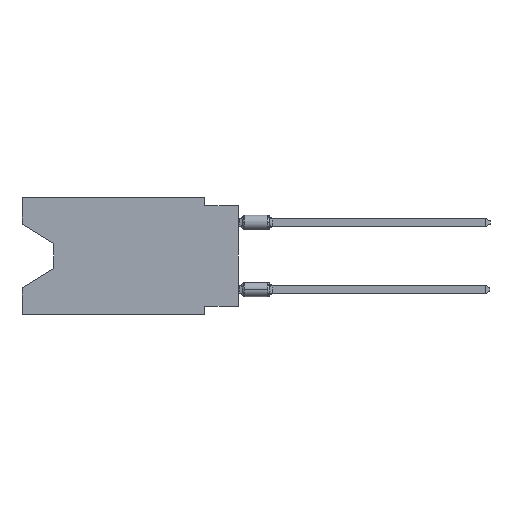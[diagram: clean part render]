
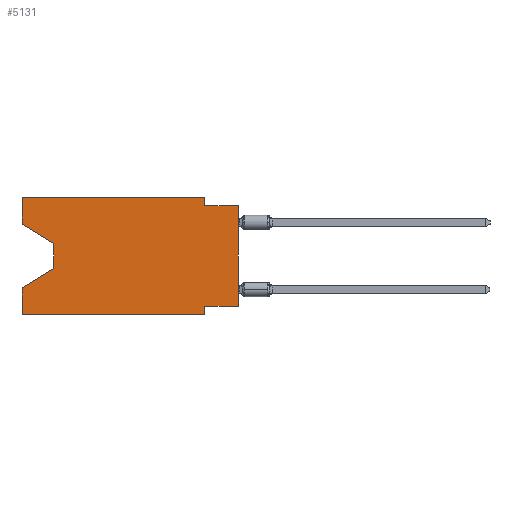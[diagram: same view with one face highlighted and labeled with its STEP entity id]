
A CAD part, left-side view. The second image highlights one B-rep face of the part: STEP entity #5131.
In plain terms, the highlighted planar face has unit normal (-1, 0, 0).
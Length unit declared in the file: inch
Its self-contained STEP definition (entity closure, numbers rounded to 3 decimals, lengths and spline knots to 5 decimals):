
#167 = VERTEX_POINT ( 'NONE', #13119 ) ;
#175 = CARTESIAN_POINT ( 'NONE',  ( 0., 0.55, -0.212 ) ) ;
#440 = EDGE_CURVE ( 'NONE', #2682, #5523, #7974, .T. ) ;
#651 = DIRECTION ( 'NONE',  ( 0., -1., 0. ) ) ;
#668 = VECTOR ( 'NONE', #1532, 39.37008 ) ;
#888 = ORIENTED_EDGE ( 'NONE', *, *, #7094, .T. ) ;
#942 = EDGE_CURVE ( 'NONE', #1382, #167, #12874, .T. ) ;
#992 = AXIS2_PLACEMENT_3D ( 'NONE', #11688, #10639, #1176 ) ;
#1126 = LINE ( 'NONE', #6563, #8957 ) ;
#1139 = ORIENTED_EDGE ( 'NONE', *, *, #942, .F. ) ;
#1176 = DIRECTION ( 'NONE',  ( 0., 0., -1. ) ) ;
#1268 = CARTESIAN_POINT ( 'NONE',  ( 0., 0.645, -0.35 ) ) ;
#1359 = CARTESIAN_POINT ( 'NONE',  ( 0., 0.1, -0.35 ) ) ;
#1382 = VERTEX_POINT ( 'NONE', #2612 ) ;
#1401 = VERTEX_POINT ( 'NONE', #12295 ) ;
#1532 = DIRECTION ( 'NONE',  ( 0., -1., 0. ) ) ;
#1541 = VECTOR ( 'NONE', #3650, 39.37008 ) ;
#1674 = DIRECTION ( 'NONE',  ( 0., 0., -1. ) ) ;
#1854 = ORIENTED_EDGE ( 'NONE', *, *, #4886, .T. ) ;
#1978 = ORIENTED_EDGE ( 'NONE', *, *, #6322, .F. ) ;
#2308 = VERTEX_POINT ( 'NONE', #2576 ) ;
#2365 = VECTOR ( 'NONE', #3681, 39.37008 ) ;
#2500 = CARTESIAN_POINT ( 'NONE',  ( 0., 0., -0.025 ) ) ;
#2503 = LINE ( 'NONE', #8784, #2365 ) ;
#2576 = CARTESIAN_POINT ( 'NONE',  ( 0., 0.55, -0.138 ) ) ;
#2612 = CARTESIAN_POINT ( 'NONE',  ( 0., 0.645, 0. ) ) ;
#2636 = DIRECTION ( 'NONE',  ( 0., -0.855, -0.519 ) ) ;
#2682 = VERTEX_POINT ( 'NONE', #1268 ) ;
#2880 = EDGE_CURVE ( 'NONE', #167, #10988, #10022, .T. ) ;
#2907 = EDGE_CURVE ( 'NONE', #9970, #5523, #13082, .T. ) ;
#3005 = CARTESIAN_POINT ( 'NONE',  ( 0., 0., -0.025 ) ) ;
#3046 = LINE ( 'NONE', #7107, #8913 ) ;
#3388 = CARTESIAN_POINT ( 'NONE',  ( 0., 0.645, 0. ) ) ;
#3650 = DIRECTION ( 'NONE',  ( 0., -1., 0. ) ) ;
#3681 = DIRECTION ( 'NONE',  ( 0., 0., -1. ) ) ;
#3987 = VERTEX_POINT ( 'NONE', #2500 ) ;
#4210 = EDGE_LOOP ( 'NONE', ( #888, #6647, #1854, #5149, #9001, #7618, #4676, #7232, #8996, #10984, #1139, #1978 ) ) ;
#4544 = VECTOR ( 'NONE', #5279, 39.37008 ) ;
#4676 = ORIENTED_EDGE ( 'NONE', *, *, #11320, .F. ) ;
#4796 = CARTESIAN_POINT ( 'NONE',  ( 0., 0.55, -0.212 ) ) ;
#4886 = EDGE_CURVE ( 'NONE', #6422, #8089, #7685, .T. ) ;
#5061 = EDGE_CURVE ( 'NONE', #11012, #3987, #3046, .T. ) ;
#5131 = ADVANCED_FACE ( 'NONE', ( #9665 ), #6404, .F. ) ;
#5149 = ORIENTED_EDGE ( 'NONE', *, *, #12013, .F. ) ;
#5279 = DIRECTION ( 'NONE',  ( 0., 0., 1. ) ) ;
#5523 = VERTEX_POINT ( 'NONE', #1359 ) ;
#5727 = LINE ( 'NONE', #7864, #11079 ) ;
#5821 = VECTOR ( 'NONE', #6702, 39.37008 ) ;
#6211 = CARTESIAN_POINT ( 'NONE',  ( 0., 0., -0.325 ) ) ;
#6322 = EDGE_CURVE ( 'NONE', #1401, #1382, #11880, .T. ) ;
#6404 = PLANE ( 'NONE',  #992 ) ;
#6422 = VERTEX_POINT ( 'NONE', #4796 ) ;
#6563 = CARTESIAN_POINT ( 'NONE',  ( 0., 0.645, -0.08025 ) ) ;
#6647 = ORIENTED_EDGE ( 'NONE', *, *, #9694, .T. ) ;
#6702 = DIRECTION ( 'NONE',  ( 0., 0., -1. ) ) ;
#6717 = VECTOR ( 'NONE', #1674, 39.37008 ) ;
#7094 = EDGE_CURVE ( 'NONE', #1401, #2308, #1126, .T. ) ;
#7107 = CARTESIAN_POINT ( 'NONE',  ( 0., 0., 0. ) ) ;
#7232 = ORIENTED_EDGE ( 'NONE', *, *, #5061, .T. ) ;
#7554 = VECTOR ( 'NONE', #8860, 39.37008 ) ;
#7597 = VECTOR ( 'NONE', #10817, 39.37008 ) ;
#7618 = ORIENTED_EDGE ( 'NONE', *, *, #2907, .F. ) ;
#7685 = LINE ( 'NONE', #175, #7597 ) ;
#7737 = CARTESIAN_POINT ( 'NONE',  ( 0., 0.1, 0. ) ) ;
#7864 = CARTESIAN_POINT ( 'NONE',  ( 0., 0., -0.325 ) ) ;
#7888 = LINE ( 'NONE', #11090, #7554 ) ;
#7974 = LINE ( 'NONE', #12299, #1541 ) ;
#8089 = VERTEX_POINT ( 'NONE', #13503 ) ;
#8094 = EDGE_CURVE ( 'NONE', #10988, #3987, #12470, .T. ) ;
#8784 = CARTESIAN_POINT ( 'NONE',  ( 0., 0.55, -0.138 ) ) ;
#8860 = DIRECTION ( 'NONE',  ( 0., 0., 1. ) ) ;
#8913 = VECTOR ( 'NONE', #12380, 39.37008 ) ;
#8957 = VECTOR ( 'NONE', #2636, 39.37008 ) ;
#8996 = ORIENTED_EDGE ( 'NONE', *, *, #8094, .F. ) ;
#9001 = ORIENTED_EDGE ( 'NONE', *, *, #440, .T. ) ;
#9665 = FACE_OUTER_BOUND ( 'NONE', #4210, .T. ) ;
#9694 = EDGE_CURVE ( 'NONE', #2308, #6422, #2503, .T. ) ;
#9735 = DIRECTION ( 'NONE',  ( 0., 1., 0. ) ) ;
#9970 = VERTEX_POINT ( 'NONE', #12038 ) ;
#10022 = LINE ( 'NONE', #7737, #5821 ) ;
#10639 = DIRECTION ( 'NONE',  ( 1., 0., 0. ) ) ;
#10817 = DIRECTION ( 'NONE',  ( 0., 0.855, -0.519 ) ) ;
#10836 = CARTESIAN_POINT ( 'NONE',  ( 0., 0.645, 0. ) ) ;
#10945 = VECTOR ( 'NONE', #651, 39.37008 ) ;
#10984 = ORIENTED_EDGE ( 'NONE', *, *, #2880, .F. ) ;
#10988 = VERTEX_POINT ( 'NONE', #12460 ) ;
#11012 = VERTEX_POINT ( 'NONE', #6211 ) ;
#11071 = CARTESIAN_POINT ( 'NONE',  ( 0., 0.1, -0.35 ) ) ;
#11079 = VECTOR ( 'NONE', #9735, 39.37008 ) ;
#11090 = CARTESIAN_POINT ( 'NONE',  ( 0., 0.645, 0. ) ) ;
#11320 = EDGE_CURVE ( 'NONE', #11012, #9970, #5727, .T. ) ;
#11688 = CARTESIAN_POINT ( 'NONE',  ( 0., 0.645, 0. ) ) ;
#11880 = LINE ( 'NONE', #10836, #4544 ) ;
#12013 = EDGE_CURVE ( 'NONE', #2682, #8089, #7888, .T. ) ;
#12038 = CARTESIAN_POINT ( 'NONE',  ( 0., 0.1, -0.325 ) ) ;
#12295 = CARTESIAN_POINT ( 'NONE',  ( 0., 0.645, -0.08025 ) ) ;
#12299 = CARTESIAN_POINT ( 'NONE',  ( 0., 0.645, -0.35 ) ) ;
#12380 = DIRECTION ( 'NONE',  ( 0., 0., 1. ) ) ;
#12460 = CARTESIAN_POINT ( 'NONE',  ( 0., 0.1, -0.025 ) ) ;
#12470 = LINE ( 'NONE', #3005, #10945 ) ;
#12874 = LINE ( 'NONE', #3388, #668 ) ;
#13082 = LINE ( 'NONE', #11071, #6717 ) ;
#13119 = CARTESIAN_POINT ( 'NONE',  ( 0., 0.1, 0. ) ) ;
#13503 = CARTESIAN_POINT ( 'NONE',  ( 0., 0.645, -0.26975 ) ) ;
